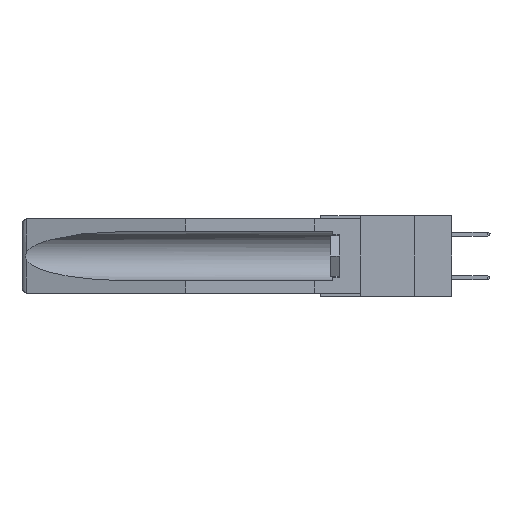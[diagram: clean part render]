
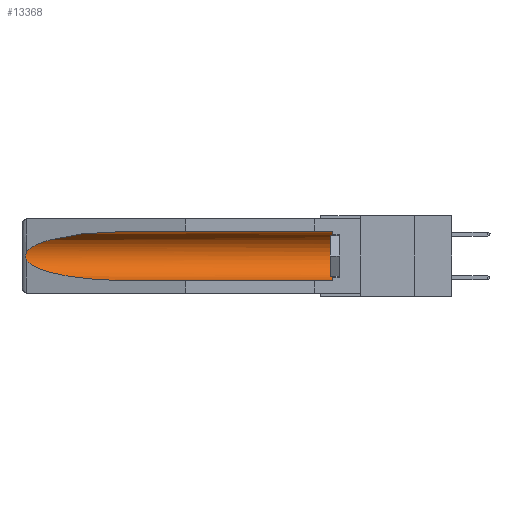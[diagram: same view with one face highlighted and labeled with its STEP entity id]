
A CAD part, left-side view. The second image highlights one B-rep face of the part: STEP entity #13368.
In plain terms, the highlighted cylindrical face has radius 2.857 mm (diameter 5.715 mm), a partial arc.
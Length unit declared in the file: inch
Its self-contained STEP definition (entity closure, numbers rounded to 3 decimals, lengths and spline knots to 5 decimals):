
#129 = LINE ( 'NONE', #25843, #10326 ) ;
#483 = EDGE_CURVE ( 'NONE', #6566, #20591, #12352, .T. ) ;
#800 = CARTESIAN_POINT ( 'NONE',  ( 0.155, 0.126, -0.1715 ) ) ;
#920 = CARTESIAN_POINT ( 'NONE',  ( 0.26537, 1.52718, -0.19328 ) ) ;
#1081 = CARTESIAN_POINT ( 'NONE',  ( 0.155, 1.07973, -0.284 ) ) ;
#1736 = CARTESIAN_POINT ( 'NONE',  ( 0.26537, 1.52718, -0.14972 ) ) ;
#1841 = CARTESIAN_POINT ( 'NONE',  ( 0.2673, 1.5327, -0.16383 ) ) ;
#2102 = CARTESIAN_POINT ( 'NONE',  ( 0.21114, 1.30732, -0.284 ) ) ;
#2838 =( BOUNDED_CURVE ( )  B_SPLINE_CURVE ( 3, ( #11433, #23115, #13753, #22716 ),
 .UNSPECIFIED., .F., .F. ) 
 B_SPLINE_CURVE_WITH_KNOTS ( ( 4, 4 ),
 ( 4.71239, 6.08839 ),
 .UNSPECIFIED. ) 
 CURVE ( )  GEOMETRIC_REPRESENTATION_ITEM ( )  RATIONAL_B_SPLINE_CURVE ( ( 1., 0.848, 0.848, 1. ) ) 
 REPRESENTATION_ITEM ( '' )  );
#3334 = ORIENTED_EDGE ( 'NONE', *, *, #6021, .T. ) ;
#3870 = CARTESIAN_POINT ( 'NONE',  ( 0.26597, 1.52961, -0.15275 ) ) ;
#4436 = CARTESIAN_POINT ( 'NONE',  ( 0.155, 1.07973, -0.284 ) ) ;
#5153 = CYLINDRICAL_SURFACE ( 'NONE', #19281, 0.1125 ) ;
#5517 = CARTESIAN_POINT ( 'NONE',  ( 0.26537, 1.52718, -0.14972 ) ) ;
#5590 = AXIS2_PLACEMENT_3D ( 'NONE', #800, #17048, #19404 ) ;
#6021 = EDGE_CURVE ( 'NONE', #14164, #27510, #2838, .T. ) ;
#6228 = CARTESIAN_POINT ( 'NONE',  ( 0.2675, 1.53308, -0.17534 ) ) ;
#6434 = CARTESIAN_POINT ( 'NONE',  ( 0.155, 0.126, -0.059 ) ) ;
#6534 = CARTESIAN_POINT ( 'NONE',  ( 0.26655, 1.53094, -0.18657 ) ) ;
#6566 = VERTEX_POINT ( 'NONE', #6923 ) ;
#6577 = LINE ( 'NONE', #9352, #11999 ) ;
#6923 = CARTESIAN_POINT ( 'NONE',  ( 0.155, 0.126, -0.284 ) ) ;
#7278 = VERTEX_POINT ( 'NONE', #1081 ) ;
#8862 = CARTESIAN_POINT ( 'NONE',  ( 0.26537, 1.52718, -0.19328 ) ) ;
#9224 = EDGE_CURVE ( 'NONE', #27510, #20346, #23913, .T. ) ;
#9319 = CARTESIAN_POINT ( 'NONE',  ( 0.26537, 1.52718, -0.19328 ) ) ;
#9352 = CARTESIAN_POINT ( 'NONE',  ( 0.155, -0.30754, -0.059 ) ) ;
#9399 = DIRECTION ( 'NONE',  ( 0., 1., 0. ) ) ;
#10326 = VECTOR ( 'NONE', #9399, 39.37008 ) ;
#11110 = EDGE_CURVE ( 'NONE', #6566, #7278, #129, .T. ) ;
#11126 = ORIENTED_EDGE ( 'NONE', *, *, #19233, .T. ) ;
#11433 = CARTESIAN_POINT ( 'NONE',  ( 0.155, 1.07973, -0.059 ) ) ;
#11999 = VECTOR ( 'NONE', #21239, 39.37008 ) ;
#12352 = CIRCLE ( 'NONE', #5590, 0.1125 ) ;
#12759 = FACE_OUTER_BOUND ( 'NONE', #21078, .T. ) ;
#13368 = ADVANCED_FACE ( 'NONE', ( #12759 ), #5153, .F. ) ;
#13753 = CARTESIAN_POINT ( 'NONE',  ( 0.25451, 1.48313, -0.09465 ) ) ;
#13879 = EDGE_CURVE ( 'NONE', #20591, #14164, #6577, .T. ) ;
#14164 = VERTEX_POINT ( 'NONE', #29114 ) ;
#14876 = DIRECTION ( 'NONE',  ( 0., 0., 1. ) ) ;
#15165 = CARTESIAN_POINT ( 'NONE',  ( 0.155, -0.30754, -0.1715 ) ) ;
#17048 = DIRECTION ( 'NONE',  ( 0., -1., 0. ) ) ;
#18111 = CARTESIAN_POINT ( 'NONE',  ( 0.2673, 1.53269, -0.17917 ) ) ;
#19233 = EDGE_CURVE ( 'NONE', #20346, #7278, #21702, .T. ) ;
#19281 = AXIS2_PLACEMENT_3D ( 'NONE', #15165, #29085, #14876 ) ;
#19404 = DIRECTION ( 'NONE',  ( 0., 0., 1. ) ) ;
#20154 = CARTESIAN_POINT ( 'NONE',  ( 0.2675, 1.53308, -0.16763 ) ) ;
#20346 = VERTEX_POINT ( 'NONE', #920 ) ;
#20591 = VERTEX_POINT ( 'NONE', #6434 ) ;
#21078 = EDGE_LOOP ( 'NONE', ( #3334, #28469, #11126, #25334, #24084, #28900 ) ) ;
#21239 = DIRECTION ( 'NONE',  ( 0., 1., 0. ) ) ;
#21702 =( BOUNDED_CURVE ( )  B_SPLINE_CURVE ( 3, ( #9319, #25641, #2102, #4436 ),
 .UNSPECIFIED., .F., .F. ) 
 B_SPLINE_CURVE_WITH_KNOTS ( ( 4, 4 ),
 ( 0.1948, 1.5708 ),
 .UNSPECIFIED. ) 
 CURVE ( )  GEOMETRIC_REPRESENTATION_ITEM ( )  RATIONAL_B_SPLINE_CURVE ( ( 1., 0.848, 0.848, 1. ) ) 
 REPRESENTATION_ITEM ( '' )  );
#22716 = CARTESIAN_POINT ( 'NONE',  ( 0.26537, 1.52718, -0.14972 ) ) ;
#22774 = CARTESIAN_POINT ( 'NONE',  ( 0.26597, 1.5296, -0.19026 ) ) ;
#23115 = CARTESIAN_POINT ( 'NONE',  ( 0.21114, 1.30732, -0.059 ) ) ;
#23913 = B_SPLINE_CURVE_WITH_KNOTS ( 'NONE', 3,
 ( #1736, #3870, #27305, #1841, #20154, #6228, #18111, #6534, #22774, #8862 ),
 .UNSPECIFIED., .F., .F.,
 ( 4, 2, 2, 2, 4 ),
 ( 0., 0.00029, 0.00058, 0.00087, 0.00117 ),
 .UNSPECIFIED. ) ;
#24084 = ORIENTED_EDGE ( 'NONE', *, *, #483, .T. ) ;
#25334 = ORIENTED_EDGE ( 'NONE', *, *, #11110, .F. ) ;
#25641 = CARTESIAN_POINT ( 'NONE',  ( 0.25451, 1.48313, -0.24835 ) ) ;
#25843 = CARTESIAN_POINT ( 'NONE',  ( 0.155, -0.30754, -0.284 ) ) ;
#27305 = CARTESIAN_POINT ( 'NONE',  ( 0.26654, 1.53092, -0.15636 ) ) ;
#27510 = VERTEX_POINT ( 'NONE', #5517 ) ;
#28469 = ORIENTED_EDGE ( 'NONE', *, *, #9224, .T. ) ;
#28900 = ORIENTED_EDGE ( 'NONE', *, *, #13879, .T. ) ;
#29085 = DIRECTION ( 'NONE',  ( 0., 1., 0. ) ) ;
#29114 = CARTESIAN_POINT ( 'NONE',  ( 0.155, 1.07973, -0.059 ) ) ;
